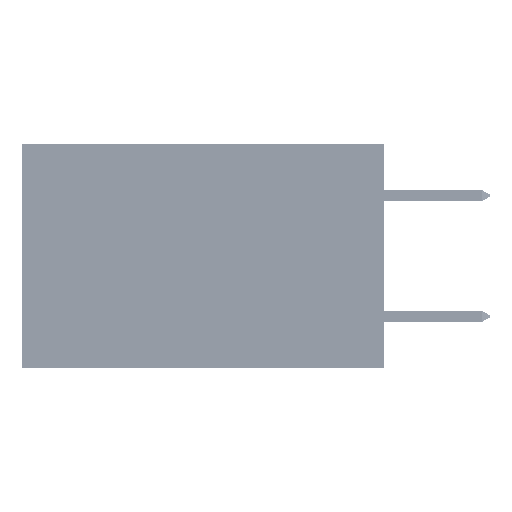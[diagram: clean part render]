
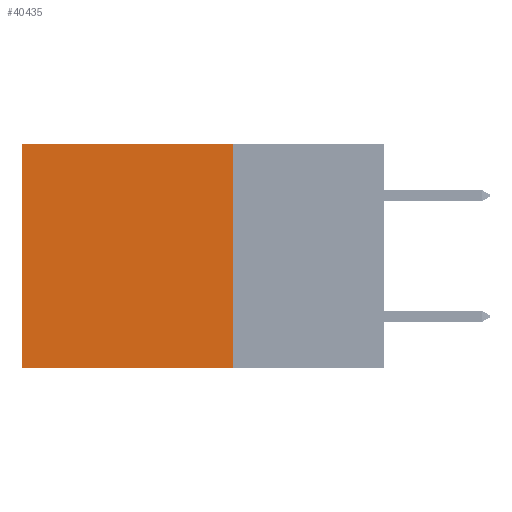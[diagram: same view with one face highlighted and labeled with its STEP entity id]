
A CAD part, left-side view. The second image highlights one B-rep face of the part: STEP entity #40435.
In plain terms, the highlighted planar face has unit normal (-1, 0, 0).
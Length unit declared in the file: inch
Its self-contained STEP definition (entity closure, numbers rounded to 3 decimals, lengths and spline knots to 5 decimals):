
#2822 = CARTESIAN_POINT ( 'NONE',  ( 0.2875, 0.25, -0.37 ) ) ;
#2840 = LINE ( 'NONE', #20402, #8029 ) ;
#4158 = FACE_OUTER_BOUND ( 'NONE', #17780, .T. ) ;
#4238 = ORIENTED_EDGE ( 'NONE', *, *, #35690, .F. ) ;
#5627 = CARTESIAN_POINT ( 'NONE',  ( 0.2875, 0.25, 0. ) ) ;
#5871 = LINE ( 'NONE', #8830, #51385 ) ;
#8029 = VECTOR ( 'NONE', #37671, 39.37008 ) ;
#8830 = CARTESIAN_POINT ( 'NONE',  ( 0.2875, 0.25, 0. ) ) ;
#9624 = VERTEX_POINT ( 'NONE', #20410 ) ;
#17780 = EDGE_LOOP ( 'NONE', ( #27974, #27086, #4238, #38140 ) ) ;
#17909 = DIRECTION ( 'NONE',  ( 1., 0., 0. ) ) ;
#20402 = CARTESIAN_POINT ( 'NONE',  ( 0.2875, 0.25, -0.37 ) ) ;
#20410 = CARTESIAN_POINT ( 'NONE',  ( 0.2875, 0.6, 0. ) ) ;
#21690 = CARTESIAN_POINT ( 'NONE',  ( 0.2875, 0.6, 0. ) ) ;
#22289 = DIRECTION ( 'NONE',  ( 0., 0., -1. ) ) ;
#22395 = EDGE_CURVE ( 'NONE', #9624, #39248, #38346, .T. ) ;
#24979 = AXIS2_PLACEMENT_3D ( 'NONE', #43006, #17909, #22289 ) ;
#27086 = ORIENTED_EDGE ( 'NONE', *, *, #49873, .F. ) ;
#27202 = CARTESIAN_POINT ( 'NONE',  ( 0.2875, 0.6, -0.37 ) ) ;
#27974 = ORIENTED_EDGE ( 'NONE', *, *, #22395, .T. ) ;
#27982 = EDGE_CURVE ( 'NONE', #43233, #9624, #5871, .T. ) ;
#28830 = CARTESIAN_POINT ( 'NONE',  ( 0.2875, 0.25, 0. ) ) ;
#29709 = VERTEX_POINT ( 'NONE', #2822 ) ;
#30621 = DIRECTION ( 'NONE',  ( 0., 0., -1. ) ) ;
#32344 = LINE ( 'NONE', #5627, #39496 ) ;
#35690 = EDGE_CURVE ( 'NONE', #43233, #29709, #32344, .T. ) ;
#36401 = VECTOR ( 'NONE', #30621, 39.37008 ) ;
#37671 = DIRECTION ( 'NONE',  ( 0., 1., 0. ) ) ;
#38140 = ORIENTED_EDGE ( 'NONE', *, *, #27982, .T. ) ;
#38346 = LINE ( 'NONE', #21690, #36401 ) ;
#38461 = PLANE ( 'NONE',  #24979 ) ;
#38719 = DIRECTION ( 'NONE',  ( 0., 0., -1. ) ) ;
#39248 = VERTEX_POINT ( 'NONE', #27202 ) ;
#39496 = VECTOR ( 'NONE', #38719, 39.37008 ) ;
#40435 = ADVANCED_FACE ( 'NONE', ( #4158 ), #38461, .F. ) ;
#43006 = CARTESIAN_POINT ( 'NONE',  ( 0.2875, 0.25, 0. ) ) ;
#43233 = VERTEX_POINT ( 'NONE', #28830 ) ;
#49181 = DIRECTION ( 'NONE',  ( 0., 1., 0. ) ) ;
#49873 = EDGE_CURVE ( 'NONE', #29709, #39248, #2840, .T. ) ;
#51385 = VECTOR ( 'NONE', #49181, 39.37008 ) ;
